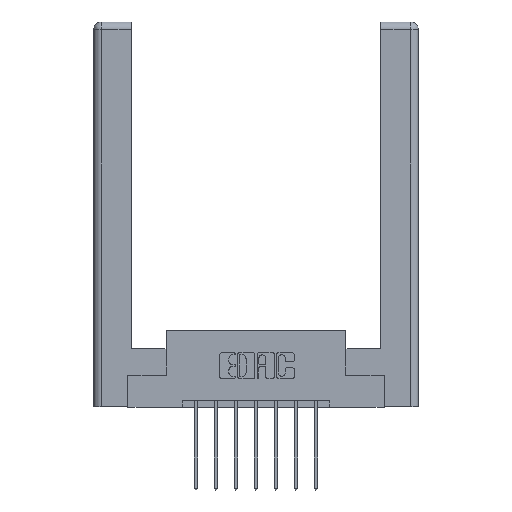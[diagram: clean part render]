
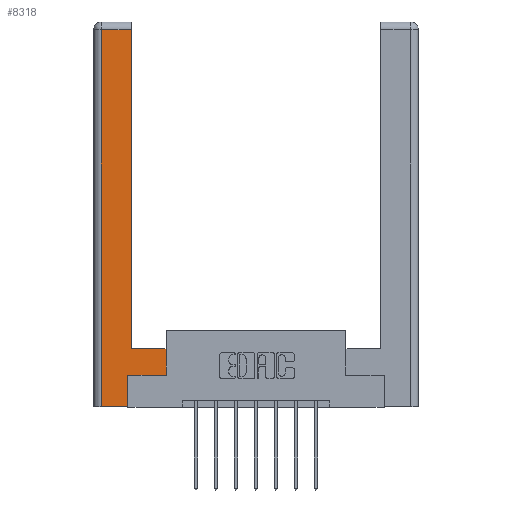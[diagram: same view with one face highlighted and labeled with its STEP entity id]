
A CAD part, top view. The second image highlights one B-rep face of the part: STEP entity #8318.
In plain terms, the highlighted planar face has unit normal (0, 0, 1).
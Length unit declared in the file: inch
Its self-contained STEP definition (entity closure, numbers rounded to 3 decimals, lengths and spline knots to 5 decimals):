
#111 = CARTESIAN_POINT ( 'NONE',  ( 0.295, 2.94, 0. ) ) ;
#120 = CARTESIAN_POINT ( 'NONE',  ( 0.565, 0.245, 0. ) ) ;
#279 = EDGE_CURVE ( 'NONE', #12115, #12034, #2941, .T. ) ;
#559 = DIRECTION ( 'NONE',  ( 0., -1., 0. ) ) ;
#785 = VECTOR ( 'NONE', #10442, 39.37008 ) ;
#974 = VECTOR ( 'NONE', #559, 39.37008 ) ;
#1115 = EDGE_CURVE ( 'NONE', #5588, #6389, #5227, .T. ) ;
#1118 = CARTESIAN_POINT ( 'NONE',  ( 0.565, 0.245, 0. ) ) ;
#1374 = VECTOR ( 'NONE', #5950, 39.37008 ) ;
#1637 = EDGE_CURVE ( 'NONE', #6389, #7837, #12355, .T. ) ;
#1929 = EDGE_CURVE ( 'NONE', #7837, #10742, #11903, .T. ) ;
#2250 = EDGE_CURVE ( 'NONE', #12034, #5588, #4251, .T. ) ;
#2356 = FACE_OUTER_BOUND ( 'NONE', #10787, .T. ) ;
#2941 = LINE ( 'NONE', #8499, #785 ) ;
#3593 = EDGE_CURVE ( 'NONE', #4908, #6437, #4654, .T. ) ;
#3720 = DIRECTION ( 'NONE',  ( 0., 0., -1. ) ) ;
#3976 = CARTESIAN_POINT ( 'NONE',  ( 0.265, 0.245, 0. ) ) ;
#4040 = ORIENTED_EDGE ( 'NONE', *, *, #2250, .T. ) ;
#4251 = LINE ( 'NONE', #5041, #6988 ) ;
#4654 = LINE ( 'NONE', #10409, #10139 ) ;
#4745 = PLANE ( 'NONE',  #8951 ) ;
#4908 = VERTEX_POINT ( 'NONE', #111 ) ;
#5041 = CARTESIAN_POINT ( 'NONE',  ( 0.265, 0.245, 0. ) ) ;
#5227 = LINE ( 'NONE', #120, #1374 ) ;
#5280 = EDGE_CURVE ( 'NONE', #6437, #12115, #6041, .T. ) ;
#5588 = VERTEX_POINT ( 'NONE', #3976 ) ;
#5950 = DIRECTION ( 'NONE',  ( 1., 0., 0. ) ) ;
#6041 = LINE ( 'NONE', #10129, #974 ) ;
#6349 = ORIENTED_EDGE ( 'NONE', *, *, #3593, .T. ) ;
#6389 = VERTEX_POINT ( 'NONE', #1118 ) ;
#6437 = VERTEX_POINT ( 'NONE', #7711 ) ;
#6556 = VECTOR ( 'NONE', #10142, 39.37008 ) ;
#6720 = CARTESIAN_POINT ( 'NONE',  ( 0.265, 0., 0. ) ) ;
#6988 = VECTOR ( 'NONE', #8983, 39.37008 ) ;
#7119 = EDGE_CURVE ( 'NONE', #10742, #4908, #8017, .T. ) ;
#7168 = CARTESIAN_POINT ( 'NONE',  ( 0.295, 3., 0. ) ) ;
#7412 = ORIENTED_EDGE ( 'NONE', *, *, #7119, .T. ) ;
#7602 = CARTESIAN_POINT ( 'NONE',  ( 0.295, 0.45, 0. ) ) ;
#7663 = CARTESIAN_POINT ( 'NONE',  ( 0., 0., 0. ) ) ;
#7711 = CARTESIAN_POINT ( 'NONE',  ( 0.0615, 2.94, 0. ) ) ;
#7837 = VERTEX_POINT ( 'NONE', #11689 ) ;
#8017 = LINE ( 'NONE', #7168, #9065 ) ;
#8318 = ADVANCED_FACE ( 'NONE', ( #2356 ), #4745, .F. ) ;
#8499 = CARTESIAN_POINT ( 'NONE',  ( 0.265, 0., 0. ) ) ;
#8594 = DIRECTION ( 'NONE',  ( -1., 0., 0. ) ) ;
#8676 = ORIENTED_EDGE ( 'NONE', *, *, #1115, .T. ) ;
#8951 = AXIS2_PLACEMENT_3D ( 'NONE', #7663, #3720, #10538 ) ;
#8983 = DIRECTION ( 'NONE',  ( 0., 1., 0. ) ) ;
#9065 = VECTOR ( 'NONE', #10157, 39.37008 ) ;
#9498 = ORIENTED_EDGE ( 'NONE', *, *, #5280, .T. ) ;
#9982 = CARTESIAN_POINT ( 'NONE',  ( 0.565, 0.45, 0. ) ) ;
#10128 = ORIENTED_EDGE ( 'NONE', *, *, #279, .T. ) ;
#10129 = CARTESIAN_POINT ( 'NONE',  ( 0.0615, 0., 0. ) ) ;
#10139 = VECTOR ( 'NONE', #8594, 39.37008 ) ;
#10142 = DIRECTION ( 'NONE',  ( 0., 1., 0. ) ) ;
#10157 = DIRECTION ( 'NONE',  ( 0., 1., 0. ) ) ;
#10409 = CARTESIAN_POINT ( 'NONE',  ( 0.0615, 2.94, 0. ) ) ;
#10442 = DIRECTION ( 'NONE',  ( 1., 0., 0. ) ) ;
#10538 = DIRECTION ( 'NONE',  ( -1., 0., 0. ) ) ;
#10742 = VERTEX_POINT ( 'NONE', #11246 ) ;
#10787 = EDGE_LOOP ( 'NONE', ( #7412, #6349, #9498, #10128, #4040, #8676, #12031, #12435 ) ) ;
#11246 = CARTESIAN_POINT ( 'NONE',  ( 0.295, 0.45, 0. ) ) ;
#11556 = DIRECTION ( 'NONE',  ( -1., 0., 0. ) ) ;
#11689 = CARTESIAN_POINT ( 'NONE',  ( 0.565, 0.45, 0. ) ) ;
#11764 = CARTESIAN_POINT ( 'NONE',  ( 0.0615, 0., 0. ) ) ;
#11903 = LINE ( 'NONE', #7602, #12489 ) ;
#12031 = ORIENTED_EDGE ( 'NONE', *, *, #1637, .T. ) ;
#12034 = VERTEX_POINT ( 'NONE', #6720 ) ;
#12115 = VERTEX_POINT ( 'NONE', #11764 ) ;
#12355 = LINE ( 'NONE', #9982, #6556 ) ;
#12435 = ORIENTED_EDGE ( 'NONE', *, *, #1929, .T. ) ;
#12489 = VECTOR ( 'NONE', #11556, 39.37008 ) ;
